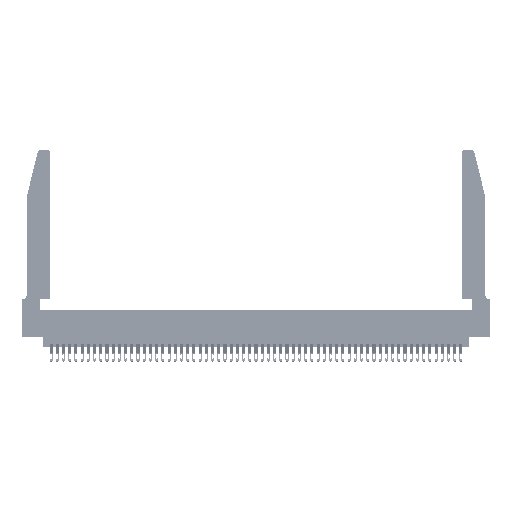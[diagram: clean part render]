
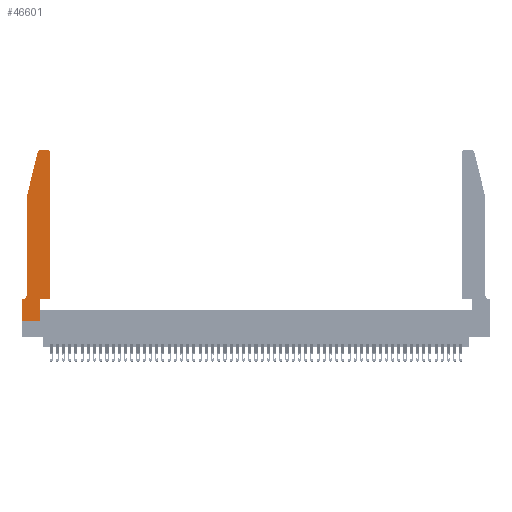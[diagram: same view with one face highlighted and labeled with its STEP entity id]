
A CAD part, top view. The second image highlights one B-rep face of the part: STEP entity #46601.
In plain terms, the highlighted planar face has unit normal (0, 0, 1).
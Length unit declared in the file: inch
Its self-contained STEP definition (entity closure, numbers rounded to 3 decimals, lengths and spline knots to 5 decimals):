
#54 = LINE ( 'NONE', #49903, #27694 ) ;
#110 = CIRCLE ( 'NONE', #53937, 0.07 ) ;
#994 = CARTESIAN_POINT ( 'NONE',  ( 0.4205, 2.75, 0.37 ) ) ;
#1225 = VECTOR ( 'NONE', #44589, 39.37008 ) ;
#1294 = EDGE_CURVE ( 'NONE', #30195, #7268, #36804, .T. ) ;
#2395 = VERTEX_POINT ( 'NONE', #994 ) ;
#2679 = VERTEX_POINT ( 'NONE', #23286 ) ;
#2843 = VERTEX_POINT ( 'NONE', #24914 ) ;
#3776 = EDGE_CURVE ( 'NONE', #7268, #2679, #31250, .T. ) ;
#6438 = VECTOR ( 'NONE', #9051, 39.37008 ) ;
#6940 = VERTEX_POINT ( 'NONE', #40977 ) ;
#7204 = VERTEX_POINT ( 'NONE', #26599 ) ;
#7268 = VERTEX_POINT ( 'NONE', #39467 ) ;
#7618 = ORIENTED_EDGE ( 'NONE', *, *, #12945, .T. ) ;
#7923 = LINE ( 'NONE', #11424, #51321 ) ;
#8623 = EDGE_CURVE ( 'NONE', #38890, #2395, #38756, .T. ) ;
#9051 = DIRECTION ( 'NONE',  ( -1., 0., 0. ) ) ;
#9881 = LINE ( 'NONE', #16447, #53870 ) ;
#10417 = CARTESIAN_POINT ( 'NONE',  ( 0.4505, 0.35, 0.37 ) ) ;
#10822 = CARTESIAN_POINT ( 'NONE',  ( 0.4205, 2.72, 0.37 ) ) ;
#11069 = VERTEX_POINT ( 'NONE', #47946 ) ;
#11424 = CARTESIAN_POINT ( 'NONE',  ( 0., 0., 0.37 ) ) ;
#11475 = VERTEX_POINT ( 'NONE', #46433 ) ;
#12186 = DIRECTION ( 'NONE',  ( 0., -1., 0. ) ) ;
#12264 = EDGE_CURVE ( 'NONE', #20891, #38890, #32407, .T. ) ;
#12363 = AXIS2_PLACEMENT_3D ( 'NONE', #10822, #15046, #48301 ) ;
#12945 = EDGE_CURVE ( 'NONE', #7204, #11069, #7923, .T. ) ;
#13556 = CARTESIAN_POINT ( 'NONE',  ( 0.0055, 0.42, 0.37 ) ) ;
#14371 = ORIENTED_EDGE ( 'NONE', *, *, #39809, .T. ) ;
#15046 = DIRECTION ( 'NONE',  ( 0., 0., 1. ) ) ;
#15366 = LINE ( 'NONE', #20302, #35787 ) ;
#16425 = VERTEX_POINT ( 'NONE', #48719 ) ;
#16447 = CARTESIAN_POINT ( 'NONE',  ( 0.0755, 2., 0.37 ) ) ;
#17435 = ORIENTED_EDGE ( 'NONE', *, *, #12264, .T. ) ;
#17889 = EDGE_CURVE ( 'NONE', #2679, #6940, #9881, .T. ) ;
#18995 = EDGE_LOOP ( 'NONE', ( #36914, #21464, #40648, #41464, #21094, #14371, #36587, #7618, #28800, #22726, #17435, #45106 ) ) ;
#20302 = CARTESIAN_POINT ( 'NONE',  ( 0., 0., 0.37 ) ) ;
#20891 = VERTEX_POINT ( 'NONE', #40355 ) ;
#21094 = ORIENTED_EDGE ( 'NONE', *, *, #46740, .T. ) ;
#21464 = ORIENTED_EDGE ( 'NONE', *, *, #1294, .T. ) ;
#21851 = DIRECTION ( 'NONE',  ( 0., 0., -1. ) ) ;
#22296 = CARTESIAN_POINT ( 'NONE',  ( 0.4505, 0.35, 0.37 ) ) ;
#22726 = ORIENTED_EDGE ( 'NONE', *, *, #50653, .T. ) ;
#23286 = CARTESIAN_POINT ( 'NONE',  ( 0.0755, 2., 0.37 ) ) ;
#23474 = DIRECTION ( 'NONE',  ( 0., 0., 1. ) ) ;
#24742 = DIRECTION ( 'NONE',  ( -1., 0., 0. ) ) ;
#24914 = CARTESIAN_POINT ( 'NONE',  ( 0.2865, 0.35, 0.37 ) ) ;
#26599 = CARTESIAN_POINT ( 'NONE',  ( 0., 0., 0.37 ) ) ;
#26832 = AXIS2_PLACEMENT_3D ( 'NONE', #42443, #41899, #50890 ) ;
#27524 = DIRECTION ( 'NONE',  ( 1., 0., 0. ) ) ;
#27694 = VECTOR ( 'NONE', #24742, 39.37008 ) ;
#28041 = EDGE_CURVE ( 'NONE', #11069, #2843, #36650, .T. ) ;
#28218 = DIRECTION ( 'NONE',  ( -0.239, -0.971, 0. ) ) ;
#28800 = ORIENTED_EDGE ( 'NONE', *, *, #28041, .T. ) ;
#29757 = VECTOR ( 'NONE', #51689, 39.37008 ) ;
#30195 = VERTEX_POINT ( 'NONE', #43207 ) ;
#30210 = LINE ( 'NONE', #10417, #1225 ) ;
#30221 = CARTESIAN_POINT ( 'NONE',  ( 0.0755, 0.35, 0.37 ) ) ;
#30518 = DIRECTION ( 'NONE',  ( -1., 0., 0. ) ) ;
#31250 = LINE ( 'NONE', #44723, #33859 ) ;
#32407 = LINE ( 'NONE', #22296, #29757 ) ;
#33341 = VECTOR ( 'NONE', #37352, 39.37008 ) ;
#33526 = CARTESIAN_POINT ( 'NONE',  ( 0.2865, 0.35, 0.37 ) ) ;
#33859 = VECTOR ( 'NONE', #28218, 39.37008 ) ;
#35787 = VECTOR ( 'NONE', #53945, 39.37008 ) ;
#36536 = CARTESIAN_POINT ( 'NONE',  ( 0.4505, 2.72, 0.37 ) ) ;
#36587 = ORIENTED_EDGE ( 'NONE', *, *, #43037, .T. ) ;
#36650 = LINE ( 'NONE', #33526, #33341 ) ;
#36728 = LINE ( 'NONE', #30221, #6438 ) ;
#36804 = CIRCLE ( 'NONE', #38995, 0.03 ) ;
#36914 = ORIENTED_EDGE ( 'NONE', *, *, #47215, .T. ) ;
#37352 = DIRECTION ( 'NONE',  ( 0., 1., 0. ) ) ;
#38756 = CIRCLE ( 'NONE', #12363, 0.03 ) ;
#38890 = VERTEX_POINT ( 'NONE', #36536 ) ;
#38995 = AXIS2_PLACEMENT_3D ( 'NONE', #52696, #23474, #27524 ) ;
#39467 = CARTESIAN_POINT ( 'NONE',  ( 0.25487, 2.72718, 0.37 ) ) ;
#39809 = EDGE_CURVE ( 'NONE', #11475, #16425, #36728, .T. ) ;
#40355 = CARTESIAN_POINT ( 'NONE',  ( 0.4505, 0.35, 0.37 ) ) ;
#40648 = ORIENTED_EDGE ( 'NONE', *, *, #3776, .T. ) ;
#40977 = CARTESIAN_POINT ( 'NONE',  ( 0.0755, 0.42, 0.37 ) ) ;
#41032 = DIRECTION ( 'NONE',  ( 1., 0., 0. ) ) ;
#41464 = ORIENTED_EDGE ( 'NONE', *, *, #17889, .T. ) ;
#41899 = DIRECTION ( 'NONE',  ( 0., 0., 1. ) ) ;
#42443 = CARTESIAN_POINT ( 'NONE',  ( 0., 0.35, 0.37 ) ) ;
#43037 = EDGE_CURVE ( 'NONE', #16425, #7204, #15366, .T. ) ;
#43207 = CARTESIAN_POINT ( 'NONE',  ( 0.284, 2.75, 0.37 ) ) ;
#44589 = DIRECTION ( 'NONE',  ( 1., 0., 0. ) ) ;
#44723 = CARTESIAN_POINT ( 'NONE',  ( 0.0755, 2., 0.37 ) ) ;
#45106 = ORIENTED_EDGE ( 'NONE', *, *, #8623, .T. ) ;
#46433 = CARTESIAN_POINT ( 'NONE',  ( 0.0055, 0.35, 0.37 ) ) ;
#46601 = ADVANCED_FACE ( 'NONE', ( #54047 ), #54449, .T. ) ;
#46740 = EDGE_CURVE ( 'NONE', #6940, #11475, #110, .T. ) ;
#47215 = EDGE_CURVE ( 'NONE', #2395, #30195, #54, .T. ) ;
#47946 = CARTESIAN_POINT ( 'NONE',  ( 0.2865, 0., 0.37 ) ) ;
#48301 = DIRECTION ( 'NONE',  ( 1., 0., 0. ) ) ;
#48719 = CARTESIAN_POINT ( 'NONE',  ( 0., 0.35, 0.37 ) ) ;
#49903 = CARTESIAN_POINT ( 'NONE',  ( 0.2605, 2.75, 0.37 ) ) ;
#50653 = EDGE_CURVE ( 'NONE', #2843, #20891, #30210, .T. ) ;
#50890 = DIRECTION ( 'NONE',  ( 1., 0., 0. ) ) ;
#51321 = VECTOR ( 'NONE', #41032, 39.37008 ) ;
#51689 = DIRECTION ( 'NONE',  ( 0., 1., 0. ) ) ;
#52696 = CARTESIAN_POINT ( 'NONE',  ( 0.284, 2.72, 0.37 ) ) ;
#53870 = VECTOR ( 'NONE', #12186, 39.37008 ) ;
#53937 = AXIS2_PLACEMENT_3D ( 'NONE', #13556, #21851, #30518 ) ;
#53945 = DIRECTION ( 'NONE',  ( 0., -1., 0. ) ) ;
#54047 = FACE_OUTER_BOUND ( 'NONE', #18995, .T. ) ;
#54449 = PLANE ( 'NONE',  #26832 ) ;
